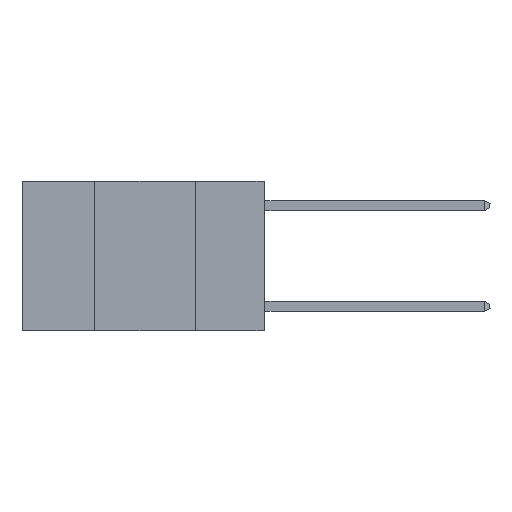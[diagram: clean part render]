
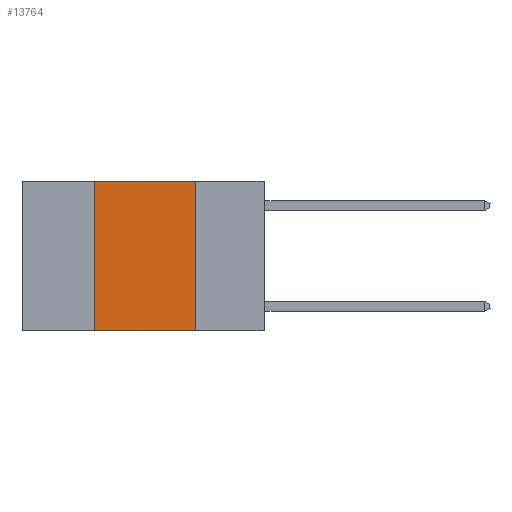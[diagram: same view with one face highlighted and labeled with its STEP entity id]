
A CAD part, left-side view. The second image highlights one B-rep face of the part: STEP entity #13764.
In plain terms, the highlighted planar face has unit normal (-1, 0, 0).
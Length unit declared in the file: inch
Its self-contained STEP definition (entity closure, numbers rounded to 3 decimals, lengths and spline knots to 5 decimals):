
#1000 = VECTOR ( 'NONE', #19765, 39.37008 ) ;
#1075 = CARTESIAN_POINT ( 'NONE',  ( 0., 0.17, 0. ) ) ;
#2317 = FACE_OUTER_BOUND ( 'NONE', #19001, .T. ) ;
#3977 = EDGE_CURVE ( 'NONE', #17881, #18088, #11928, .T. ) ;
#4240 = PLANE ( 'NONE',  #14491 ) ;
#4348 = DIRECTION ( 'NONE',  ( 1., 0., 0. ) ) ;
#4464 = VERTEX_POINT ( 'NONE', #5231 ) ;
#4603 = CARTESIAN_POINT ( 'NONE',  ( 0., 0.6, -0.37 ) ) ;
#5231 = CARTESIAN_POINT ( 'NONE',  ( 0., 0.42, -0.37 ) ) ;
#5969 = ORIENTED_EDGE ( 'NONE', *, *, #18143, .F. ) ;
#6334 = CARTESIAN_POINT ( 'NONE',  ( 0., 0.42, 0. ) ) ;
#8531 = DIRECTION ( 'NONE',  ( 0., 0., -1. ) ) ;
#8594 = EDGE_CURVE ( 'NONE', #20824, #17881, #23176, .T. ) ;
#9946 = VECTOR ( 'NONE', #8531, 39.37008 ) ;
#10192 = CARTESIAN_POINT ( 'NONE',  ( 0., 0.6, 0. ) ) ;
#10529 = ORIENTED_EDGE ( 'NONE', *, *, #3977, .F. ) ;
#10606 = CARTESIAN_POINT ( 'NONE',  ( 0., 0.17, -0.37 ) ) ;
#11873 = DIRECTION ( 'NONE',  ( 0., 0., -1. ) ) ;
#11928 = LINE ( 'NONE', #19344, #9946 ) ;
#12141 = DIRECTION ( 'NONE',  ( 0., -1., 0. ) ) ;
#13764 = ADVANCED_FACE ( 'NONE', ( #2317 ), #4240, .F. ) ;
#14491 = AXIS2_PLACEMENT_3D ( 'NONE', #20978, #4348, #11873 ) ;
#15661 = DIRECTION ( 'NONE',  ( 0., 0., 1. ) ) ;
#16037 = CARTESIAN_POINT ( 'NONE',  ( 0., 0.42, 0. ) ) ;
#16909 = EDGE_CURVE ( 'NONE', #4464, #18088, #19655, .T. ) ;
#17881 = VERTEX_POINT ( 'NONE', #1075 ) ;
#18088 = VERTEX_POINT ( 'NONE', #10606 ) ;
#18143 = EDGE_CURVE ( 'NONE', #4464, #20824, #21241, .T. ) ;
#19001 = EDGE_LOOP ( 'NONE', ( #10529, #19978, #5969, #20333 ) ) ;
#19344 = CARTESIAN_POINT ( 'NONE',  ( 0., 0.17, 0. ) ) ;
#19655 = LINE ( 'NONE', #4603, #1000 ) ;
#19765 = DIRECTION ( 'NONE',  ( 0., -1., 0. ) ) ;
#19978 = ORIENTED_EDGE ( 'NONE', *, *, #8594, .F. ) ;
#20083 = VECTOR ( 'NONE', #12141, 39.37008 ) ;
#20333 = ORIENTED_EDGE ( 'NONE', *, *, #16909, .T. ) ;
#20824 = VERTEX_POINT ( 'NONE', #16037 ) ;
#20978 = CARTESIAN_POINT ( 'NONE',  ( 0., 0.6, 0. ) ) ;
#21241 = LINE ( 'NONE', #6334, #22284 ) ;
#22284 = VECTOR ( 'NONE', #15661, 39.37008 ) ;
#23176 = LINE ( 'NONE', #10192, #20083 ) ;
